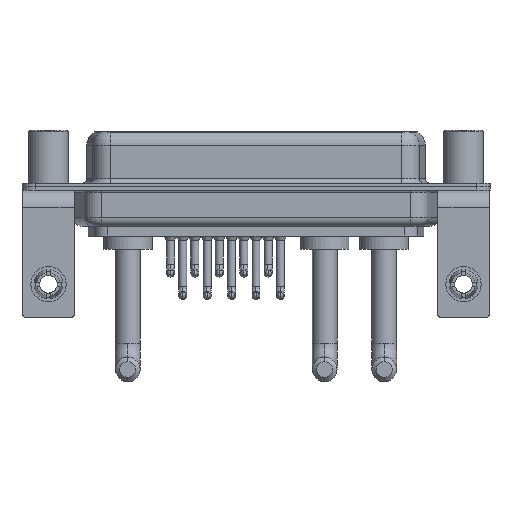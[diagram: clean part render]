
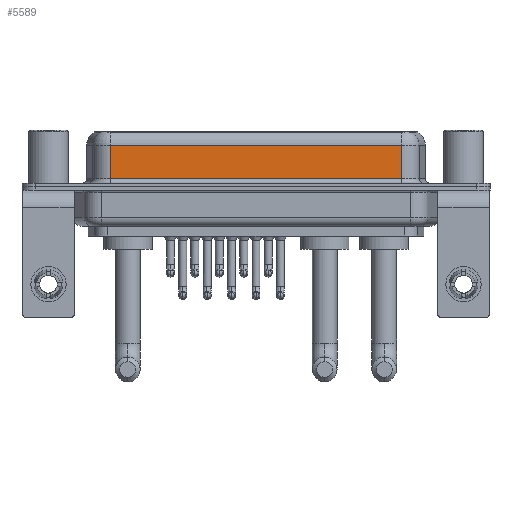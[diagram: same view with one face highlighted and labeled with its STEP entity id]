
A CAD part, front view. The second image highlights one B-rep face of the part: STEP entity #5589.
In plain terms, the highlighted planar face has unit normal (0, -1, 0).
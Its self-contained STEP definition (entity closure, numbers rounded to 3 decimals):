
#1624 = VECTOR ( 'NONE', #4969, 1000. ) ;
#1868 = CARTESIAN_POINT ( 'NONE',  ( 40.037, -3.95, 0.9 ) ) ;
#2130 = CARTESIAN_POINT ( 'NONE',  ( 7.013, -3.95, 0.9 ) ) ;
#2708 = DIRECTION ( 'NONE',  ( -1., 0., 0. ) ) ;
#3278 = PLANE ( 'NONE',  #4961 ) ;
#3386 = DIRECTION ( 'NONE',  ( 0., 1., 0. ) ) ;
#3958 = EDGE_CURVE ( 'NONE', #6736, #8120, #12548, .T. ) ;
#3963 = ORIENTED_EDGE ( 'NONE', *, *, #19143, .T. ) ;
#4223 = EDGE_CURVE ( 'NONE', #17420, #8120, #22469, .T. ) ;
#4631 = DIRECTION ( 'NONE',  ( 0., 0., -1. ) ) ;
#4961 = AXIS2_PLACEMENT_3D ( 'NONE', #18713, #3386, #22379 ) ;
#4969 = DIRECTION ( 'NONE',  ( 1., 0., 0. ) ) ;
#5197 = EDGE_CURVE ( 'NONE', #10947, #17420, #10825, .T. ) ;
#5589 = ADVANCED_FACE ( 'NONE', ( #19050 ), #3278, .F. ) ;
#6017 = CARTESIAN_POINT ( 'NONE',  ( 7.013, -3.95, 6.4 ) ) ;
#6736 = VERTEX_POINT ( 'NONE', #8704 ) ;
#7384 = VECTOR ( 'NONE', #2708, 1000. ) ;
#8120 = VERTEX_POINT ( 'NONE', #9492 ) ;
#8342 = ORIENTED_EDGE ( 'NONE', *, *, #4223, .T. ) ;
#8411 = EDGE_LOOP ( 'NONE', ( #21121, #3963, #17238, #8342 ) ) ;
#8704 = CARTESIAN_POINT ( 'NONE',  ( 40.037, -3.95, 4.65 ) ) ;
#9209 = DIRECTION ( 'NONE',  ( 0., 0., -1. ) ) ;
#9492 = CARTESIAN_POINT ( 'NONE',  ( 40.037, -3.95, 0.9 ) ) ;
#10825 = LINE ( 'NONE', #6017, #18116 ) ;
#10947 = VERTEX_POINT ( 'NONE', #19170 ) ;
#12548 = LINE ( 'NONE', #17903, #13333 ) ;
#13333 = VECTOR ( 'NONE', #4631, 1000. ) ;
#15070 = LINE ( 'NONE', #18373, #7384 ) ;
#17238 = ORIENTED_EDGE ( 'NONE', *, *, #5197, .T. ) ;
#17420 = VERTEX_POINT ( 'NONE', #2130 ) ;
#17903 = CARTESIAN_POINT ( 'NONE',  ( 40.037, -3.95, 6.4 ) ) ;
#18116 = VECTOR ( 'NONE', #9209, 1000. ) ;
#18373 = CARTESIAN_POINT ( 'NONE',  ( 40.037, -3.95, 4.65 ) ) ;
#18713 = CARTESIAN_POINT ( 'NONE',  ( 40.037, -3.95, 6.4 ) ) ;
#19050 = FACE_OUTER_BOUND ( 'NONE', #8411, .T. ) ;
#19143 = EDGE_CURVE ( 'NONE', #6736, #10947, #15070, .T. ) ;
#19170 = CARTESIAN_POINT ( 'NONE',  ( 7.013, -3.95, 4.65 ) ) ;
#21121 = ORIENTED_EDGE ( 'NONE', *, *, #3958, .F. ) ;
#22379 = DIRECTION ( 'NONE',  ( 0., 0., 1. ) ) ;
#22469 = LINE ( 'NONE', #1868, #1624 ) ;
